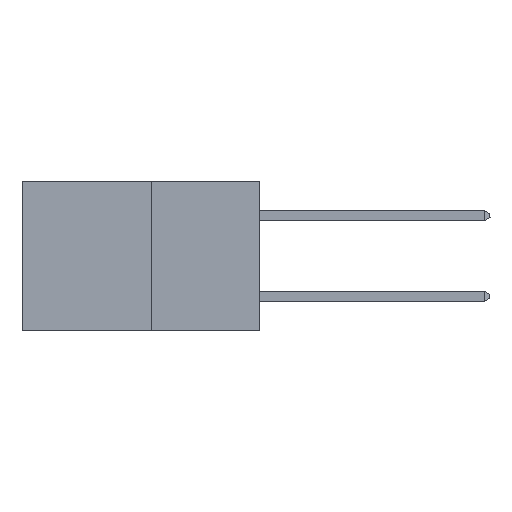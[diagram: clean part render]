
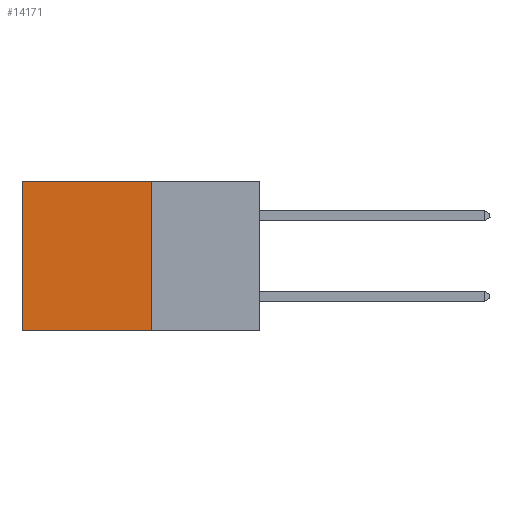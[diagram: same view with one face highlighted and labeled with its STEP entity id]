
A CAD part, left-side view. The second image highlights one B-rep face of the part: STEP entity #14171.
In plain terms, the highlighted planar face has unit normal (-1, 0, 0).
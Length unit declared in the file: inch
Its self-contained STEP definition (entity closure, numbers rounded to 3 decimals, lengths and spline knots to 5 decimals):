
#69 = DIRECTION ( 'NONE',  ( 0., 0., -1. ) ) ;
#85 = ORIENTED_EDGE ( 'NONE', *, *, #3286, .T. ) ;
#94 = DIRECTION ( 'NONE',  ( 0., 0., -1. ) ) ;
#1166 = VECTOR ( 'NONE', #6841, 39.37008 ) ;
#1804 = VECTOR ( 'NONE', #11014, 39.37008 ) ;
#2232 = AXIS2_PLACEMENT_3D ( 'NONE', #16155, #8275, #94 ) ;
#2550 = VERTEX_POINT ( 'NONE', #3447 ) ;
#2910 = EDGE_CURVE ( 'NONE', #17229, #2550, #15427, .T. ) ;
#3286 = EDGE_CURVE ( 'NONE', #2550, #4010, #16231, .T. ) ;
#3447 = CARTESIAN_POINT ( 'NONE',  ( 0.277, 0.59, 0. ) ) ;
#4010 = VERTEX_POINT ( 'NONE', #12872 ) ;
#4124 = EDGE_CURVE ( 'NONE', #17229, #7368, #8607, .T. ) ;
#4179 = VECTOR ( 'NONE', #69, 39.37008 ) ;
#5302 = CARTESIAN_POINT ( 'NONE',  ( 0.277, 0.27, 0. ) ) ;
#6145 = CARTESIAN_POINT ( 'NONE',  ( 0.277, 0.59, -0.37 ) ) ;
#6841 = DIRECTION ( 'NONE',  ( 0., 1., 0. ) ) ;
#6889 = CARTESIAN_POINT ( 'NONE',  ( 0.277, 0.27, 0. ) ) ;
#7126 = DIRECTION ( 'NONE',  ( 0., 0., -1. ) ) ;
#7368 = VERTEX_POINT ( 'NONE', #13735 ) ;
#8275 = DIRECTION ( 'NONE',  ( 1., 0., 0. ) ) ;
#8447 = ORIENTED_EDGE ( 'NONE', *, *, #2910, .T. ) ;
#8605 = LINE ( 'NONE', #9706, #1804 ) ;
#8607 = LINE ( 'NONE', #12677, #4179 ) ;
#9346 = EDGE_CURVE ( 'NONE', #7368, #4010, #8605, .T. ) ;
#9706 = CARTESIAN_POINT ( 'NONE',  ( 0.277, 0.27, -0.37 ) ) ;
#11014 = DIRECTION ( 'NONE',  ( 0., 1., 0. ) ) ;
#12197 = ORIENTED_EDGE ( 'NONE', *, *, #4124, .F. ) ;
#12368 = EDGE_LOOP ( 'NONE', ( #85, #15222, #12197, #8447 ) ) ;
#12677 = CARTESIAN_POINT ( 'NONE',  ( 0.277, 0.27, -0.37 ) ) ;
#12795 = VECTOR ( 'NONE', #7126, 39.37008 ) ;
#12872 = CARTESIAN_POINT ( 'NONE',  ( 0.277, 0.59, -0.37 ) ) ;
#13735 = CARTESIAN_POINT ( 'NONE',  ( 0.277, 0.27, -0.37 ) ) ;
#14171 = ADVANCED_FACE ( 'NONE', ( #15183 ), #14763, .F. ) ;
#14763 = PLANE ( 'NONE',  #2232 ) ;
#15183 = FACE_OUTER_BOUND ( 'NONE', #12368, .T. ) ;
#15222 = ORIENTED_EDGE ( 'NONE', *, *, #9346, .F. ) ;
#15427 = LINE ( 'NONE', #5302, #1166 ) ;
#16155 = CARTESIAN_POINT ( 'NONE',  ( 0.277, 0.27, -0.37 ) ) ;
#16231 = LINE ( 'NONE', #6145, #12795 ) ;
#17229 = VERTEX_POINT ( 'NONE', #6889 ) ;
